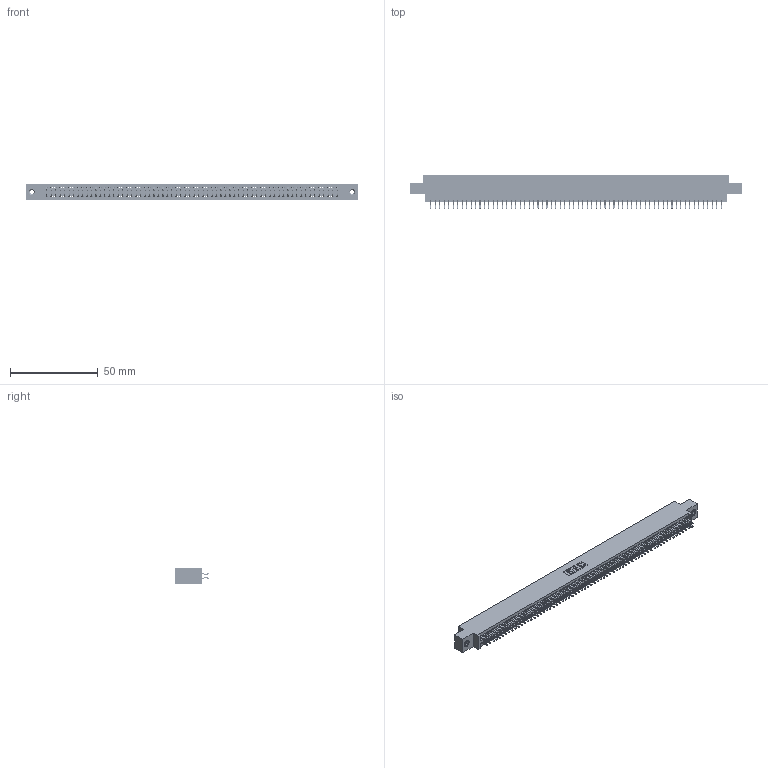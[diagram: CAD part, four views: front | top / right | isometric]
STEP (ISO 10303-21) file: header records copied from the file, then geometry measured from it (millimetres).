
FILE_DESCRIPTION (( 'STEP AP203' ), '1' );
FILE_NAME ('345-132-556-808.STEP', '2018-10-20T06:15:11', ( '' ), ( '' ), 'SwSTEP 2.0', 'SolidWorks 2016', '' );
FILE_SCHEMA (( 'CONFIG_CONTROL_DESIGN' ));
Length unit declared in the file: inch
Products named in the file (4): 345 Part_0.170 Offset - 0.156 Dia-TI; 345-250-001_345-250-003-102; 345-132-556-808; 345-292-001_556 Tail
Assembly tree (135 placements, depth 2):
  345-132-556-808
    345 Part_0.170 Offset - 0.156 Dia-TI
    345-292-001_556 Tail  x132
    345-250-001_345-250-003-102  x2
Bounding box: 188.85 x 19.24 x 9.4 mm (x, y, z)
Volume: 18442.6 mm3; surface area: 27767.5 mm2
Topology: 135 solids, 135 shells, 7582 faces, 22533 edges, 14838 vertices
Faces by surface type: plane 5000, cylinder 2566, cone 12, torus 4
Entity records: 50092 total; most frequent: CARTESIAN_POINT 8371, ORIENTED_EDGE 8286, DIRECTION 7365, EDGE_CURVE 4143, VECTOR 3719, LINE 3719, VERTEX_POINT 2756, AXIS2_PLACEMENT_3D 1823
